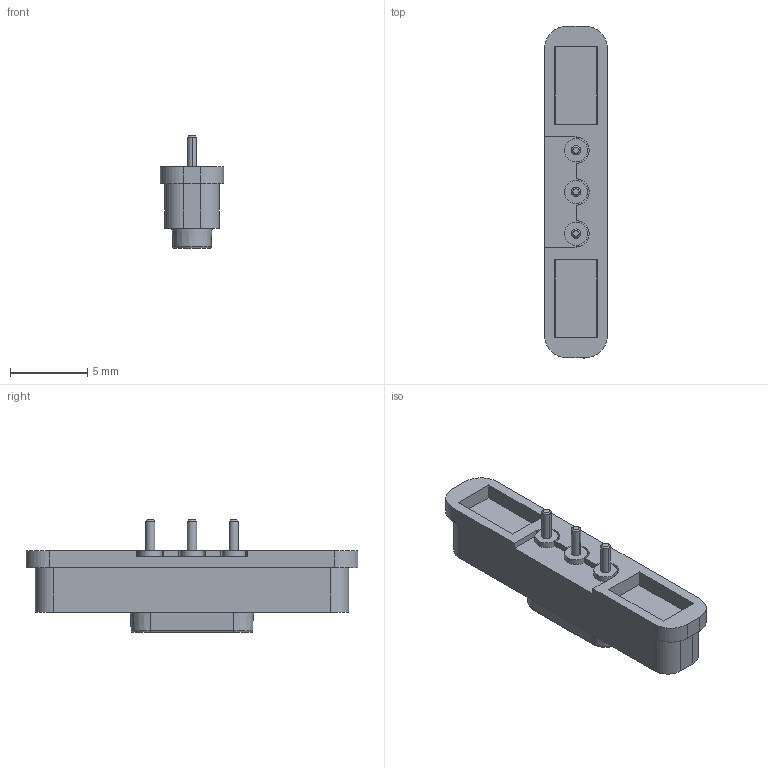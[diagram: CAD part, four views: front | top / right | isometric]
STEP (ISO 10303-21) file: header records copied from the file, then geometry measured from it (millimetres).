
FILE_DESCRIPTION (( 'STEP AP214' ), '1' );
FILE_NAME ('685E0322250110E.STEP', '2023-05-16T17:44:59', ( '' ), ( '' ), 'SwSTEP 2.0', 'SolidWorks 2020', '' );
FILE_SCHEMA (( 'AUTOMOTIVE_DESIGN' ));
Length unit declared in the file: millimetre
Products named in the file (1): 685E0322250110E
Bounding box: 4.1 x 21.5 x 7.3 mm (x, y, z)
Volume: 282.7 mm3; surface area: 511.2 mm2
Topology: 1 solids, 1 shells, 203 faces, 523 edges, 345 vertices
Faces by surface type: plane 142, cylinder 43, cone 9, bspline 6, torus 3
Entity records: 7553 total; most frequent: CARTESIAN_POINT 1234, ORIENTED_EDGE 1046, DIRECTION 1039, EDGE_CURVE 523, LINE 403, VECTOR 403, VERTEX_POINT 345, AXIS2_PLACEMENT_3D 318
